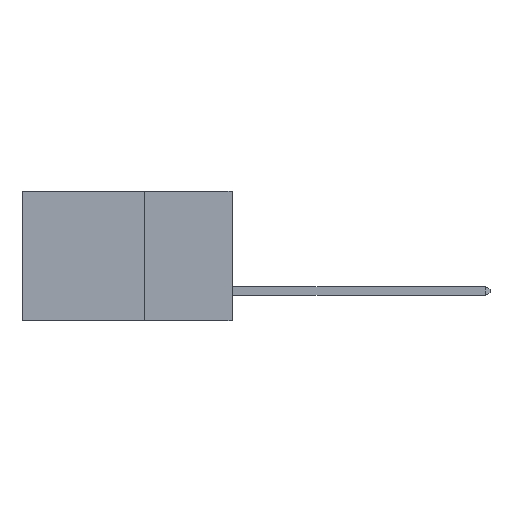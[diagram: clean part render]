
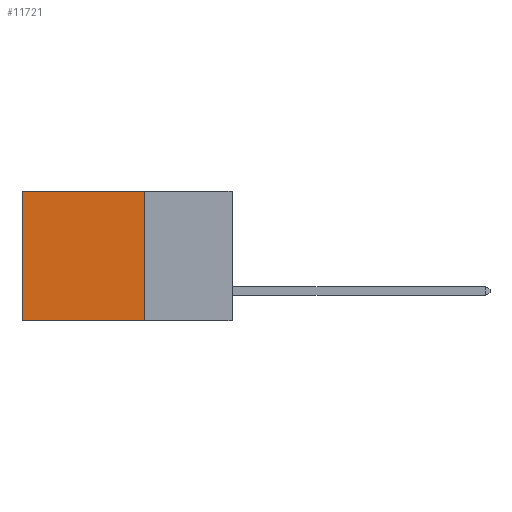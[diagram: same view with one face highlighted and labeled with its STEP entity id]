
A CAD part, left-side view. The second image highlights one B-rep face of the part: STEP entity #11721.
In plain terms, the highlighted planar face has unit normal (-1, 0, 0).
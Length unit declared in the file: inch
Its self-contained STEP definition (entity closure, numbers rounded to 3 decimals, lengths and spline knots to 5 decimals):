
#2364 = LINE ( 'NONE', #34150, #25951 ) ;
#3102 = LINE ( 'NONE', #24809, #34703 ) ;
#3142 = CARTESIAN_POINT ( 'NONE',  ( 0.2875, 0.6, -0.37 ) ) ;
#4496 = VERTEX_POINT ( 'NONE', #28088 ) ;
#7612 = EDGE_CURVE ( 'NONE', #24596, #15986, #3102, .T. ) ;
#7892 = ORIENTED_EDGE ( 'NONE', *, *, #25849, .F. ) ;
#8361 = LINE ( 'NONE', #37080, #16449 ) ;
#10142 = ORIENTED_EDGE ( 'NONE', *, *, #28279, .T. ) ;
#11593 = AXIS2_PLACEMENT_3D ( 'NONE', #29892, #11646, #32930 ) ;
#11646 = DIRECTION ( 'NONE',  ( 1., 0., 0. ) ) ;
#11721 = ADVANCED_FACE ( 'NONE', ( #20474 ), #14516, .F. ) ;
#14487 = EDGE_CURVE ( 'NONE', #20834, #15986, #2364, .T. ) ;
#14516 = PLANE ( 'NONE',  #11593 ) ;
#15656 = DIRECTION ( 'NONE',  ( 0., 1., 0. ) ) ;
#15847 = DIRECTION ( 'NONE',  ( 0., 1., 0. ) ) ;
#15986 = VERTEX_POINT ( 'NONE', #3142 ) ;
#16449 = VECTOR ( 'NONE', #15847, 39.37008 ) ;
#18178 = CARTESIAN_POINT ( 'NONE',  ( 0.2875, 0.6, 0. ) ) ;
#20389 = ORIENTED_EDGE ( 'NONE', *, *, #14487, .F. ) ;
#20474 = FACE_OUTER_BOUND ( 'NONE', #38866, .T. ) ;
#20834 = VERTEX_POINT ( 'NONE', #35267 ) ;
#24366 = CARTESIAN_POINT ( 'NONE',  ( 0.2875, 0.25, 0. ) ) ;
#24596 = VERTEX_POINT ( 'NONE', #18178 ) ;
#24809 = CARTESIAN_POINT ( 'NONE',  ( 0.2875, 0.6, 0. ) ) ;
#25849 = EDGE_CURVE ( 'NONE', #4496, #20834, #35202, .T. ) ;
#25951 = VECTOR ( 'NONE', #15656, 39.37008 ) ;
#28088 = CARTESIAN_POINT ( 'NONE',  ( 0.2875, 0.25, 0. ) ) ;
#28279 = EDGE_CURVE ( 'NONE', #4496, #24596, #8361, .T. ) ;
#29892 = CARTESIAN_POINT ( 'NONE',  ( 0.2875, 0.25, 0. ) ) ;
#32930 = DIRECTION ( 'NONE',  ( 0., 0., -1. ) ) ;
#33523 = DIRECTION ( 'NONE',  ( 0., 0., -1. ) ) ;
#33955 = DIRECTION ( 'NONE',  ( 0., 0., -1. ) ) ;
#34150 = CARTESIAN_POINT ( 'NONE',  ( 0.2875, 0.25, -0.37 ) ) ;
#34282 = VECTOR ( 'NONE', #33523, 39.37008 ) ;
#34703 = VECTOR ( 'NONE', #33955, 39.37008 ) ;
#35202 = LINE ( 'NONE', #24366, #34282 ) ;
#35267 = CARTESIAN_POINT ( 'NONE',  ( 0.2875, 0.25, -0.37 ) ) ;
#36889 = ORIENTED_EDGE ( 'NONE', *, *, #7612, .T. ) ;
#37080 = CARTESIAN_POINT ( 'NONE',  ( 0.2875, 0.25, 0. ) ) ;
#38866 = EDGE_LOOP ( 'NONE', ( #36889, #20389, #7892, #10142 ) ) ;
